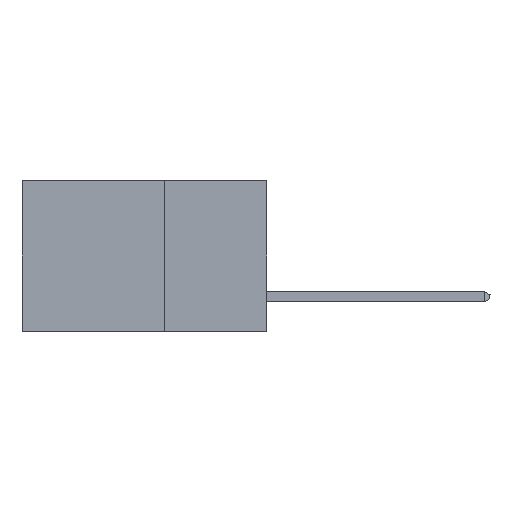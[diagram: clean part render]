
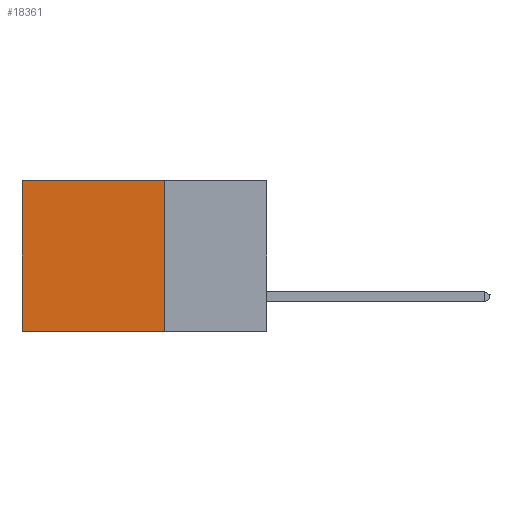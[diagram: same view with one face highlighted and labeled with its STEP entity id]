
A CAD part, left-side view. The second image highlights one B-rep face of the part: STEP entity #18361.
In plain terms, the highlighted planar face has unit normal (-1, 0, 0).
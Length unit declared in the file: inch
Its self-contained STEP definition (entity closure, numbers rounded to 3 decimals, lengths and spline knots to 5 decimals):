
#302 = ORIENTED_EDGE ( 'NONE', *, *, #5895, .T. ) ;
#1407 = VECTOR ( 'NONE', #15962, 39.37008 ) ;
#3471 = LINE ( 'NONE', #23309, #30500 ) ;
#3942 = CARTESIAN_POINT ( 'NONE',  ( 0.2875, 0.6, 0. ) ) ;
#5552 = DIRECTION ( 'NONE',  ( 0., 0., -1. ) ) ;
#5895 = EDGE_CURVE ( 'NONE', #22566, #26294, #35625, .T. ) ;
#6540 = DIRECTION ( 'NONE',  ( 1., 0., 0. ) ) ;
#7194 = CARTESIAN_POINT ( 'NONE',  ( 0.2875, 0.25, 0. ) ) ;
#8362 = DIRECTION ( 'NONE',  ( 0., 1., 0. ) ) ;
#8513 = ORIENTED_EDGE ( 'NONE', *, *, #32135, .F. ) ;
#8988 = CARTESIAN_POINT ( 'NONE',  ( 0.2875, 0.25, 0. ) ) ;
#9409 = CARTESIAN_POINT ( 'NONE',  ( 0.2875, 0.6, 0. ) ) ;
#13077 = CARTESIAN_POINT ( 'NONE',  ( 0.2875, 0.25, 0. ) ) ;
#13300 = EDGE_CURVE ( 'NONE', #26294, #19033, #15712, .T. ) ;
#13929 = EDGE_CURVE ( 'NONE', #34781, #19033, #22766, .T. ) ;
#14657 = ORIENTED_EDGE ( 'NONE', *, *, #13929, .F. ) ;
#15712 = LINE ( 'NONE', #3942, #35811 ) ;
#15962 = DIRECTION ( 'NONE',  ( 0., 1., 0. ) ) ;
#17887 = VECTOR ( 'NONE', #8362, 39.37008 ) ;
#18361 = ADVANCED_FACE ( 'NONE', ( #20748 ), #32157, .F. ) ;
#19033 = VERTEX_POINT ( 'NONE', #20825 ) ;
#20748 = FACE_OUTER_BOUND ( 'NONE', #25578, .T. ) ;
#20825 = CARTESIAN_POINT ( 'NONE',  ( 0.2875, 0.6, -0.37 ) ) ;
#21137 = DIRECTION ( 'NONE',  ( 0., 0., -1. ) ) ;
#22566 = VERTEX_POINT ( 'NONE', #13077 ) ;
#22766 = LINE ( 'NONE', #28740, #17887 ) ;
#23309 = CARTESIAN_POINT ( 'NONE',  ( 0.2875, 0.25, 0. ) ) ;
#25578 = EDGE_LOOP ( 'NONE', ( #31082, #14657, #8513, #302 ) ) ;
#26294 = VERTEX_POINT ( 'NONE', #9409 ) ;
#28740 = CARTESIAN_POINT ( 'NONE',  ( 0.2875, 0.25, -0.37 ) ) ;
#28750 = CARTESIAN_POINT ( 'NONE',  ( 0.2875, 0.25, -0.37 ) ) ;
#28994 = DIRECTION ( 'NONE',  ( 0., 0., -1. ) ) ;
#30500 = VECTOR ( 'NONE', #5552, 39.37008 ) ;
#30517 = AXIS2_PLACEMENT_3D ( 'NONE', #8988, #6540, #28994 ) ;
#31082 = ORIENTED_EDGE ( 'NONE', *, *, #13300, .T. ) ;
#32135 = EDGE_CURVE ( 'NONE', #22566, #34781, #3471, .T. ) ;
#32157 = PLANE ( 'NONE',  #30517 ) ;
#34781 = VERTEX_POINT ( 'NONE', #28750 ) ;
#35625 = LINE ( 'NONE', #7194, #1407 ) ;
#35811 = VECTOR ( 'NONE', #21137, 39.37008 ) ;
